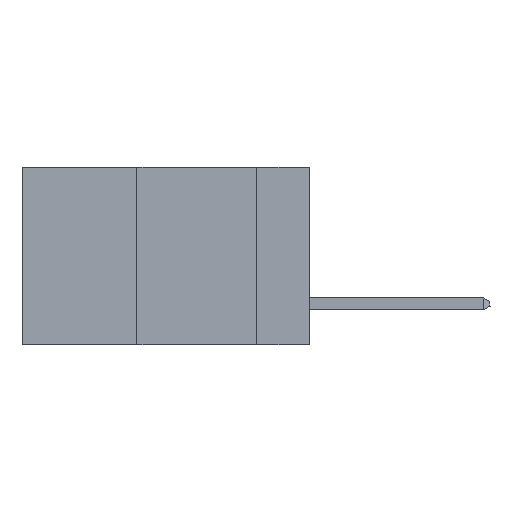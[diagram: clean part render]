
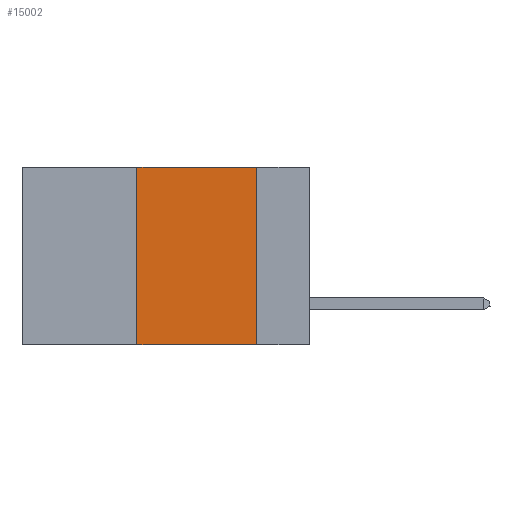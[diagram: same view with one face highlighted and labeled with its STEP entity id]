
A CAD part, left-side view. The second image highlights one B-rep face of the part: STEP entity #15002.
In plain terms, the highlighted planar face has unit normal (-1, 0, 0).
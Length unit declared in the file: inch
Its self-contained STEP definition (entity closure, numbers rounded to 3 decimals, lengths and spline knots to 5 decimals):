
#374 = DIRECTION ( 'NONE',  ( 0., -1., 0. ) ) ;
#564 = VERTEX_POINT ( 'NONE', #10668 ) ;
#1513 = CARTESIAN_POINT ( 'NONE',  ( 0., 0.11, 0. ) ) ;
#1701 = DIRECTION ( 'NONE',  ( 0., 0., -1. ) ) ;
#1970 = EDGE_LOOP ( 'NONE', ( #13686, #5513, #7792, #18071 ) ) ;
#3277 = CARTESIAN_POINT ( 'NONE',  ( 0., 0.36, 0. ) ) ;
#3497 = VECTOR ( 'NONE', #374, 39.37008 ) ;
#3763 = PLANE ( 'NONE',  #6448 ) ;
#4442 = LINE ( 'NONE', #10696, #3497 ) ;
#4712 = DIRECTION ( 'NONE',  ( 0., 0., 1. ) ) ;
#5513 = ORIENTED_EDGE ( 'NONE', *, *, #19038, .F. ) ;
#5599 = VECTOR ( 'NONE', #1701, 39.37008 ) ;
#6448 = AXIS2_PLACEMENT_3D ( 'NONE', #11016, #8300, #9535 ) ;
#7792 = ORIENTED_EDGE ( 'NONE', *, *, #9869, .F. ) ;
#7946 = LINE ( 'NONE', #1513, #5599 ) ;
#8209 = CARTESIAN_POINT ( 'NONE',  ( 0., 0.6, 0. ) ) ;
#8300 = DIRECTION ( 'NONE',  ( 1., 0., 0. ) ) ;
#8578 = VECTOR ( 'NONE', #19020, 39.37008 ) ;
#9261 = LINE ( 'NONE', #8209, #8578 ) ;
#9485 = VERTEX_POINT ( 'NONE', #11232 ) ;
#9535 = DIRECTION ( 'NONE',  ( 0., 0., -1. ) ) ;
#9869 = EDGE_CURVE ( 'NONE', #564, #16041, #15697, .T. ) ;
#10668 = CARTESIAN_POINT ( 'NONE',  ( 0., 0.36, -0.37 ) ) ;
#10696 = CARTESIAN_POINT ( 'NONE',  ( 0., 0.6, -0.37 ) ) ;
#11016 = CARTESIAN_POINT ( 'NONE',  ( 0., 0.6, 0. ) ) ;
#11232 = CARTESIAN_POINT ( 'NONE',  ( 0., 0.11, -0.37 ) ) ;
#11740 = VECTOR ( 'NONE', #4712, 39.37008 ) ;
#11861 = VERTEX_POINT ( 'NONE', #16018 ) ;
#12647 = CARTESIAN_POINT ( 'NONE',  ( 0., 0.36, 0. ) ) ;
#13011 = EDGE_CURVE ( 'NONE', #11861, #9485, #7946, .T. ) ;
#13686 = ORIENTED_EDGE ( 'NONE', *, *, #13011, .F. ) ;
#15002 = ADVANCED_FACE ( 'NONE', ( #19021 ), #3763, .F. ) ;
#15697 = LINE ( 'NONE', #12647, #11740 ) ;
#16018 = CARTESIAN_POINT ( 'NONE',  ( 0., 0.11, 0. ) ) ;
#16041 = VERTEX_POINT ( 'NONE', #3277 ) ;
#16468 = EDGE_CURVE ( 'NONE', #564, #9485, #4442, .T. ) ;
#18071 = ORIENTED_EDGE ( 'NONE', *, *, #16468, .T. ) ;
#19020 = DIRECTION ( 'NONE',  ( 0., -1., 0. ) ) ;
#19021 = FACE_OUTER_BOUND ( 'NONE', #1970, .T. ) ;
#19038 = EDGE_CURVE ( 'NONE', #16041, #11861, #9261, .T. ) ;
